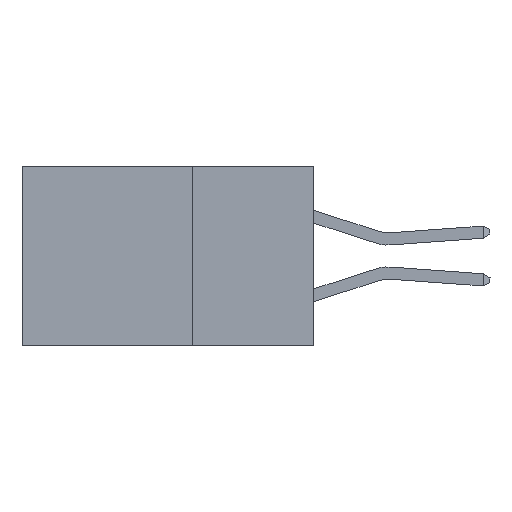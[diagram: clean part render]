
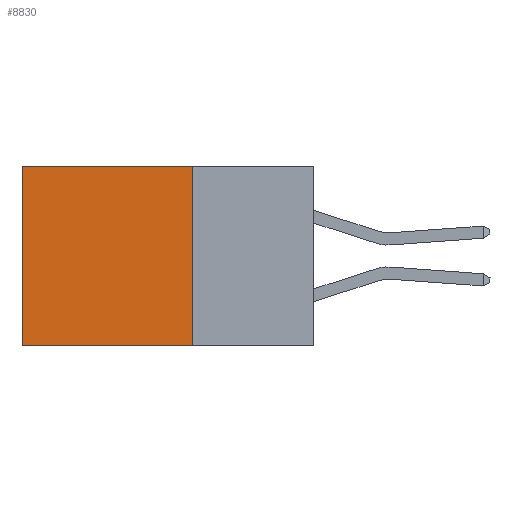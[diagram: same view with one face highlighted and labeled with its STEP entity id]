
A CAD part, left-side view. The second image highlights one B-rep face of the part: STEP entity #8830.
In plain terms, the highlighted planar face has unit normal (-1, 0, 0).
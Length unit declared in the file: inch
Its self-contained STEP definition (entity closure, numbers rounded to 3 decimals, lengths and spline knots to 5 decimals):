
#272 = LINE ( 'NONE', #391, #4393 ) ;
#317 = VERTEX_POINT ( 'NONE', #15041 ) ;
#391 = CARTESIAN_POINT ( 'NONE',  ( 0.2875, 0.25, -0.37 ) ) ;
#1178 = CARTESIAN_POINT ( 'NONE',  ( 0.2875, 0.25, 0. ) ) ;
#1412 = ORIENTED_EDGE ( 'NONE', *, *, #12101, .F. ) ;
#2628 = VERTEX_POINT ( 'NONE', #1178 ) ;
#2656 = CARTESIAN_POINT ( 'NONE',  ( 0.2875, 0.6, 0. ) ) ;
#2853 = ORIENTED_EDGE ( 'NONE', *, *, #4467, .F. ) ;
#3864 = DIRECTION ( 'NONE',  ( 0., 0., -1. ) ) ;
#4016 = DIRECTION ( 'NONE',  ( 0., 0., -1. ) ) ;
#4393 = VECTOR ( 'NONE', #13592, 39.37008 ) ;
#4467 = EDGE_CURVE ( 'NONE', #2628, #317, #11589, .T. ) ;
#4491 = CARTESIAN_POINT ( 'NONE',  ( 0.2875, 0.25, 0. ) ) ;
#4738 = FACE_OUTER_BOUND ( 'NONE', #11485, .T. ) ;
#4765 = AXIS2_PLACEMENT_3D ( 'NONE', #4861, #12288, #3864 ) ;
#4861 = CARTESIAN_POINT ( 'NONE',  ( 0.2875, 0.25, 0. ) ) ;
#8830 = ADVANCED_FACE ( 'NONE', ( #4738 ), #11967, .F. ) ;
#9303 = VECTOR ( 'NONE', #14131, 39.37008 ) ;
#9450 = VERTEX_POINT ( 'NONE', #13392 ) ;
#9676 = LINE ( 'NONE', #4491, #9303 ) ;
#11228 = VERTEX_POINT ( 'NONE', #15166 ) ;
#11485 = EDGE_LOOP ( 'NONE', ( #14514, #1412, #2853, #14015 ) ) ;
#11589 = LINE ( 'NONE', #14718, #13634 ) ;
#11967 = PLANE ( 'NONE',  #4765 ) ;
#12101 = EDGE_CURVE ( 'NONE', #317, #9450, #272, .T. ) ;
#12288 = DIRECTION ( 'NONE',  ( 1., 0., 0. ) ) ;
#12341 = LINE ( 'NONE', #2656, #14743 ) ;
#12394 = DIRECTION ( 'NONE',  ( 0., 0., -1. ) ) ;
#13345 = EDGE_CURVE ( 'NONE', #11228, #9450, #12341, .T. ) ;
#13392 = CARTESIAN_POINT ( 'NONE',  ( 0.2875, 0.6, -0.37 ) ) ;
#13592 = DIRECTION ( 'NONE',  ( 0., 1., 0. ) ) ;
#13634 = VECTOR ( 'NONE', #12394, 39.37008 ) ;
#14015 = ORIENTED_EDGE ( 'NONE', *, *, #15215, .T. ) ;
#14131 = DIRECTION ( 'NONE',  ( 0., 1., 0. ) ) ;
#14514 = ORIENTED_EDGE ( 'NONE', *, *, #13345, .T. ) ;
#14718 = CARTESIAN_POINT ( 'NONE',  ( 0.2875, 0.25, 0. ) ) ;
#14743 = VECTOR ( 'NONE', #4016, 39.37008 ) ;
#15041 = CARTESIAN_POINT ( 'NONE',  ( 0.2875, 0.25, -0.37 ) ) ;
#15166 = CARTESIAN_POINT ( 'NONE',  ( 0.2875, 0.6, 0. ) ) ;
#15215 = EDGE_CURVE ( 'NONE', #2628, #11228, #9676, .T. ) ;
